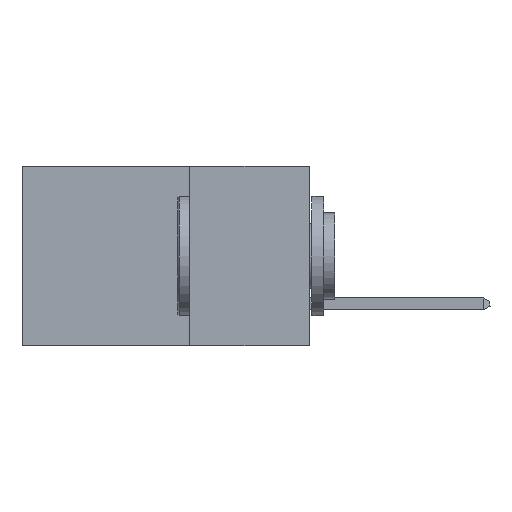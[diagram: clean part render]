
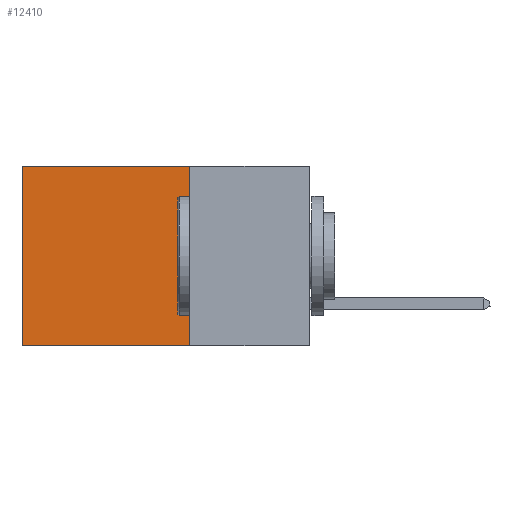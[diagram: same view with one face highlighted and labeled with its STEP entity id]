
A CAD part, left-side view. The second image highlights one B-rep face of the part: STEP entity #12410.
In plain terms, the highlighted planar face has unit normal (-1, 0, 0).
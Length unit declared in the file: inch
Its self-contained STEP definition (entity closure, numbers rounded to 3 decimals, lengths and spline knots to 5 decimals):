
#748 = VECTOR ( 'NONE', #9613, 39.37008 ) ;
#769 = ORIENTED_EDGE ( 'NONE', *, *, #6642, .T. ) ;
#787 = VERTEX_POINT ( 'NONE', #5807 ) ;
#955 = CARTESIAN_POINT ( 'NONE',  ( 0.2875, 0.6, -0.375 ) ) ;
#1089 = DIRECTION ( 'NONE',  ( 0., 0., -1. ) ) ;
#3029 = CARTESIAN_POINT ( 'NONE',  ( 0.2875, 0.25, -0.375 ) ) ;
#3036 = EDGE_LOOP ( 'NONE', ( #769, #13836, #6998, #7226 ) ) ;
#3085 = AXIS2_PLACEMENT_3D ( 'NONE', #12899, #10668, #1089 ) ;
#3235 = LINE ( 'NONE', #3029, #10932 ) ;
#3239 = LINE ( 'NONE', #13032, #748 ) ;
#3371 = EDGE_CURVE ( 'NONE', #787, #11737, #11836, .T. ) ;
#4303 = CARTESIAN_POINT ( 'NONE',  ( 0.2875, 0.25, -0.375 ) ) ;
#5226 = DIRECTION ( 'NONE',  ( 0., 0., -1. ) ) ;
#5250 = VERTEX_POINT ( 'NONE', #4303 ) ;
#5807 = CARTESIAN_POINT ( 'NONE',  ( 0.2875, 0.25, 0. ) ) ;
#6642 = EDGE_CURVE ( 'NONE', #11737, #7987, #10537, .T. ) ;
#6998 = ORIENTED_EDGE ( 'NONE', *, *, #9378, .F. ) ;
#7060 = EDGE_CURVE ( 'NONE', #5250, #7987, #3235, .T. ) ;
#7226 = ORIENTED_EDGE ( 'NONE', *, *, #3371, .T. ) ;
#7462 = DIRECTION ( 'NONE',  ( 0., 1., 0. ) ) ;
#7497 = FACE_OUTER_BOUND ( 'NONE', #3036, .T. ) ;
#7987 = VERTEX_POINT ( 'NONE', #10355 ) ;
#9378 = EDGE_CURVE ( 'NONE', #787, #5250, #3239, .T. ) ;
#9610 = DIRECTION ( 'NONE',  ( 0., 1., 0. ) ) ;
#9613 = DIRECTION ( 'NONE',  ( 0., 0., -1. ) ) ;
#9759 = PLANE ( 'NONE',  #3085 ) ;
#9929 = CARTESIAN_POINT ( 'NONE',  ( 0.2875, 0.6, 0. ) ) ;
#9991 = VECTOR ( 'NONE', #7462, 39.37008 ) ;
#10248 = VECTOR ( 'NONE', #5226, 39.37008 ) ;
#10355 = CARTESIAN_POINT ( 'NONE',  ( 0.2875, 0.6, -0.375 ) ) ;
#10537 = LINE ( 'NONE', #955, #10248 ) ;
#10668 = DIRECTION ( 'NONE',  ( 1., 0., 0. ) ) ;
#10932 = VECTOR ( 'NONE', #9610, 39.37008 ) ;
#11737 = VERTEX_POINT ( 'NONE', #9929 ) ;
#11836 = LINE ( 'NONE', #12799, #9991 ) ;
#12410 = ADVANCED_FACE ( 'NONE', ( #7497 ), #9759, .F. ) ;
#12799 = CARTESIAN_POINT ( 'NONE',  ( 0.2875, 0.25, 0. ) ) ;
#12899 = CARTESIAN_POINT ( 'NONE',  ( 0.2875, 0.25, -0.375 ) ) ;
#13032 = CARTESIAN_POINT ( 'NONE',  ( 0.2875, 0.25, -0.375 ) ) ;
#13836 = ORIENTED_EDGE ( 'NONE', *, *, #7060, .F. ) ;
